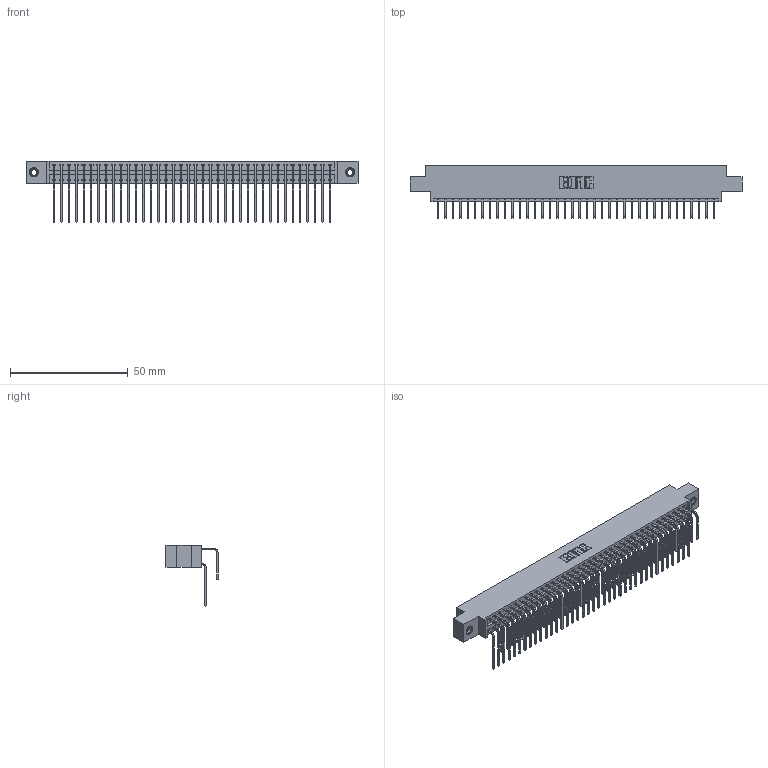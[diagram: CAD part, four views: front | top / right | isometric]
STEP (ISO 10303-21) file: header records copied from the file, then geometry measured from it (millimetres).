
FILE_DESCRIPTION (( 'STEP AP203' ), '1' );
FILE_NAME ('346-076-558-807.STEP', '2022-05-25T13:02:53', ( '' ), ( '' ), 'SwSTEP 2.0', 'SolidWorks 2020', '' );
FILE_SCHEMA (( 'CONFIG_CONTROL_DESIGN' ));
Length unit declared in the file: inch
Products named in the file (5): 345-292-001_558 Tail - 2; 346 Part_0.170 Offset - 0.156 Dia-TI; 346-076-558-807; 345-250-001_345-250-005-103; 345-292-001_558 559 Tail - 1
Assembly tree (79 placements, depth 2):
  346-076-558-807
    346 Part_0.170 Offset - 0.156 Dia-TI
    345-292-001_558 559 Tail - 1  x38
    345-292-001_558 Tail - 2  x38
    345-250-001_345-250-005-103  x2
Bounding box: 141.22 x 22.16 x 26.16 mm (x, y, z)
Volume: 14010.3 mm3; surface area: 21511.9 mm2
Topology: 79 solids, 79 shells, 4290 faces, 12713 edges, 8366 vertices
Faces by surface type: plane 2924, cylinder 1350, cone 12, torus 4
Entity records: 28440 total; most frequent: CARTESIAN_POINT 4730, ORIENTED_EDGE 4606, DIRECTION 4217, EDGE_CURVE 2303, LINE 1959, VECTOR 1959, VERTEX_POINT 1528, AXIS2_PLACEMENT_3D 1129
